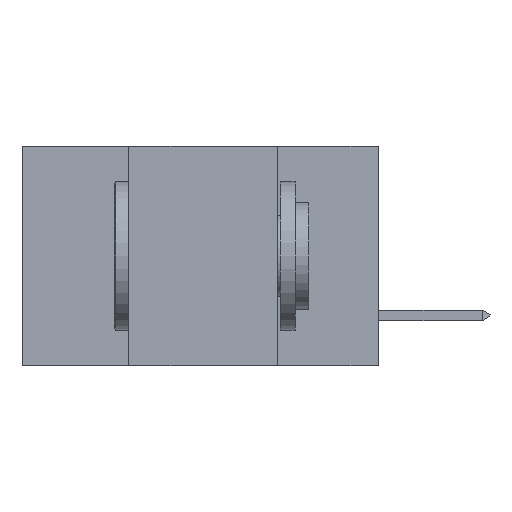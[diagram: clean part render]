
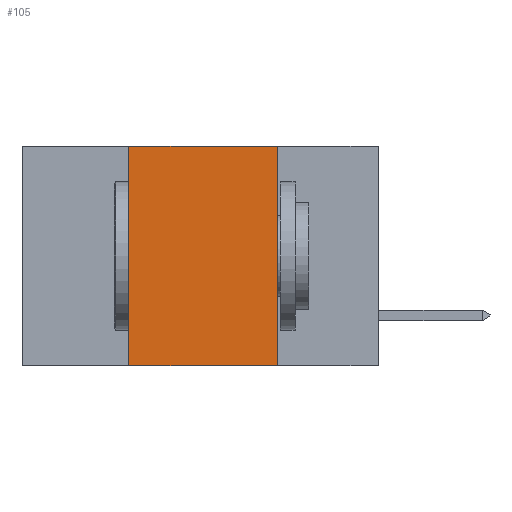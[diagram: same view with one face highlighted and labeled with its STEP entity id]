
A CAD part, left-side view. The second image highlights one B-rep face of the part: STEP entity #105.
In plain terms, the highlighted planar face has unit normal (-1, 0, 0).
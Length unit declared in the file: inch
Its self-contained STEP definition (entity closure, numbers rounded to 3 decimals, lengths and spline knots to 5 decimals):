
#105 = ADVANCED_FACE ( 'NONE', ( #1813 ), #6454, .F. ) ;
#195 = CARTESIAN_POINT ( 'NONE',  ( 0., 0.17, 0. ) ) ;
#229 = VERTEX_POINT ( 'NONE', #12817 ) ;
#1682 = ORIENTED_EDGE ( 'NONE', *, *, #7543, .T. ) ;
#1813 = FACE_OUTER_BOUND ( 'NONE', #12531, .T. ) ;
#3570 = VERTEX_POINT ( 'NONE', #13142 ) ;
#4888 = CARTESIAN_POINT ( 'NONE',  ( 0., 0.6, -0.37 ) ) ;
#5089 = VECTOR ( 'NONE', #19749, 39.37008 ) ;
#5663 = VECTOR ( 'NONE', #15919, 39.37008 ) ;
#6227 = LINE ( 'NONE', #15679, #13198 ) ;
#6454 = PLANE ( 'NONE',  #18142 ) ;
#6654 = CARTESIAN_POINT ( 'NONE',  ( 0., 0.6, 0. ) ) ;
#6887 = VECTOR ( 'NONE', #9252, 39.37008 ) ;
#7543 = EDGE_CURVE ( 'NONE', #229, #17229, #12764, .T. ) ;
#7814 = ORIENTED_EDGE ( 'NONE', *, *, #13688, .F. ) ;
#8809 = LINE ( 'NONE', #14974, #5089 ) ;
#9252 = DIRECTION ( 'NONE',  ( 0., -1., 0. ) ) ;
#9637 = DIRECTION ( 'NONE',  ( 0., 0., -1. ) ) ;
#10105 = EDGE_CURVE ( 'NONE', #3570, #20640, #17119, .T. ) ;
#11322 = ORIENTED_EDGE ( 'NONE', *, *, #10105, .F. ) ;
#12531 = EDGE_LOOP ( 'NONE', ( #16683, #11322, #7814, #1682 ) ) ;
#12637 = DIRECTION ( 'NONE',  ( 0., 0., -1. ) ) ;
#12764 = LINE ( 'NONE', #4888, #5663 ) ;
#12817 = CARTESIAN_POINT ( 'NONE',  ( 0., 0.42, -0.37 ) ) ;
#12945 = DIRECTION ( 'NONE',  ( 1., 0., 0. ) ) ;
#13142 = CARTESIAN_POINT ( 'NONE',  ( 0., 0.42, 0. ) ) ;
#13198 = VECTOR ( 'NONE', #12637, 39.37008 ) ;
#13688 = EDGE_CURVE ( 'NONE', #229, #3570, #8809, .T. ) ;
#14974 = CARTESIAN_POINT ( 'NONE',  ( 0., 0.42, -0.37 ) ) ;
#15679 = CARTESIAN_POINT ( 'NONE',  ( 0., 0.17, -0.37 ) ) ;
#15711 = CARTESIAN_POINT ( 'NONE',  ( 0., 0.6, 0. ) ) ;
#15919 = DIRECTION ( 'NONE',  ( 0., -1., 0. ) ) ;
#16683 = ORIENTED_EDGE ( 'NONE', *, *, #20042, .F. ) ;
#16972 = CARTESIAN_POINT ( 'NONE',  ( 0., 0.17, -0.37 ) ) ;
#17119 = LINE ( 'NONE', #15711, #6887 ) ;
#17229 = VERTEX_POINT ( 'NONE', #16972 ) ;
#18142 = AXIS2_PLACEMENT_3D ( 'NONE', #6654, #12945, #9637 ) ;
#19749 = DIRECTION ( 'NONE',  ( 0., 0., 1. ) ) ;
#20042 = EDGE_CURVE ( 'NONE', #20640, #17229, #6227, .T. ) ;
#20640 = VERTEX_POINT ( 'NONE', #195 ) ;
